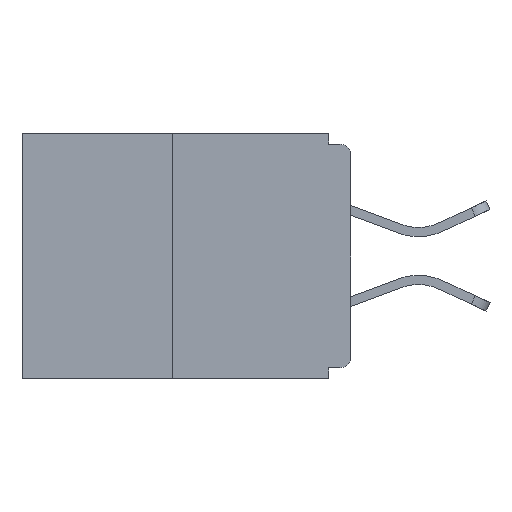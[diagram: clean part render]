
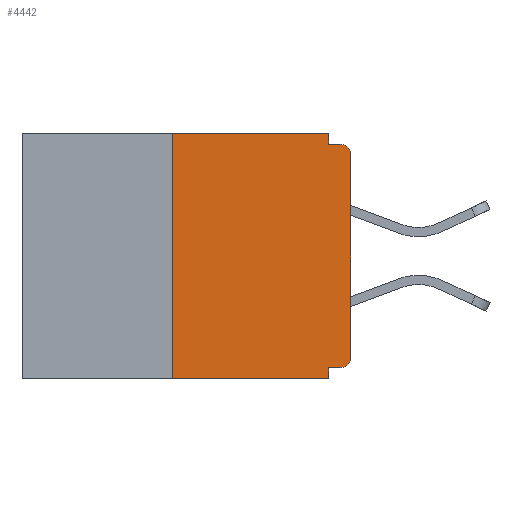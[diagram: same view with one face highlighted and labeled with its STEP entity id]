
A CAD part, left-side view. The second image highlights one B-rep face of the part: STEP entity #4442.
In plain terms, the highlighted planar face has unit normal (-1, 0, 0).
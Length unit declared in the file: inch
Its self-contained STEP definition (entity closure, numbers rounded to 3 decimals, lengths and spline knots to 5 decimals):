
#423 = CARTESIAN_POINT ( 'NONE',  ( 0., 0., -0.015 ) ) ;
#564 = VECTOR ( 'NONE', #16982, 39.37008 ) ;
#706 = DIRECTION ( 'NONE',  ( 1., 0., 0. ) ) ;
#1157 = LINE ( 'NONE', #5550, #12122 ) ;
#1200 = ORIENTED_EDGE ( 'NONE', *, *, #18923, .T. ) ;
#1649 = DIRECTION ( 'NONE',  ( 0., 0., 1. ) ) ;
#1995 = EDGE_LOOP ( 'NONE', ( #3875, #26558, #20291, #4947, #20913, #7943, #1200, #18781, #25721, #5291 ) ) ;
#2291 = DIRECTION ( 'NONE',  ( -1., 0., 0. ) ) ;
#2390 = DIRECTION ( 'NONE',  ( 0., 0., -1. ) ) ;
#3600 = DIRECTION ( 'NONE',  ( 0., -1., 0. ) ) ;
#3779 = CARTESIAN_POINT ( 'NONE',  ( 0., 0.031, -0.343 ) ) ;
#3837 = FACE_OUTER_BOUND ( 'NONE', #1995, .T. ) ;
#3875 = ORIENTED_EDGE ( 'NONE', *, *, #6598, .F. ) ;
#4348 = LINE ( 'NONE', #423, #26550 ) ;
#4442 = ADVANCED_FACE ( 'NONE', ( #3837 ), #6889, .F. ) ;
#4756 = LINE ( 'NONE', #15666, #19653 ) ;
#4944 = DIRECTION ( 'NONE',  ( 0., -1., 0. ) ) ;
#4947 = ORIENTED_EDGE ( 'NONE', *, *, #16179, .F. ) ;
#5106 = EDGE_CURVE ( 'NONE', #24350, #14958, #23606, .T. ) ;
#5291 = ORIENTED_EDGE ( 'NONE', *, *, #20488, .F. ) ;
#5550 = CARTESIAN_POINT ( 'NONE',  ( 0., 0., -0.328 ) ) ;
#5695 = CARTESIAN_POINT ( 'NONE',  ( 0., 0.031, -0.343 ) ) ;
#6598 = EDGE_CURVE ( 'NONE', #8157, #20316, #13883, .T. ) ;
#6620 = CARTESIAN_POINT ( 'NONE',  ( 0., 0., -0.03 ) ) ;
#6793 = EDGE_CURVE ( 'NONE', #8269, #20010, #9901, .T. ) ;
#6889 = PLANE ( 'NONE',  #25837 ) ;
#7943 = ORIENTED_EDGE ( 'NONE', *, *, #6793, .T. ) ;
#8157 = VERTEX_POINT ( 'NONE', #18156 ) ;
#8269 = VERTEX_POINT ( 'NONE', #18789 ) ;
#8326 = VERTEX_POINT ( 'NONE', #19890 ) ;
#8352 = CARTESIAN_POINT ( 'NONE',  ( 0., 0.031, 0. ) ) ;
#9837 = CARTESIAN_POINT ( 'NONE',  ( 0., 0.031, -0.328 ) ) ;
#9865 = VECTOR ( 'NONE', #19667, 39.37008 ) ;
#9901 = CIRCLE ( 'NONE', #16354, 0.015 ) ;
#10922 = CARTESIAN_POINT ( 'NONE',  ( 0., 0.031, 0. ) ) ;
#11319 = CARTESIAN_POINT ( 'NONE',  ( 0., 0., 0. ) ) ;
#12122 = VECTOR ( 'NONE', #13898, 39.37008 ) ;
#12250 = VECTOR ( 'NONE', #3600, 39.37008 ) ;
#12766 = CARTESIAN_POINT ( 'NONE',  ( 0., 0.015, -0.313 ) ) ;
#13309 = DIRECTION ( 'NONE',  ( 0., 0., -1. ) ) ;
#13883 = LINE ( 'NONE', #24522, #12250 ) ;
#13898 = DIRECTION ( 'NONE',  ( 0., 1., 0. ) ) ;
#14958 = VERTEX_POINT ( 'NONE', #15532 ) ;
#15428 = VECTOR ( 'NONE', #18938, 39.37008 ) ;
#15532 = CARTESIAN_POINT ( 'NONE',  ( 0., 0.015, -0.015 ) ) ;
#15666 = CARTESIAN_POINT ( 'NONE',  ( 0., 0.46, -0.343 ) ) ;
#16142 = LINE ( 'NONE', #10922, #564 ) ;
#16179 = EDGE_CURVE ( 'NONE', #23628, #19715, #21429, .T. ) ;
#16354 = AXIS2_PLACEMENT_3D ( 'NONE', #12766, #21296, #2390 ) ;
#16982 = DIRECTION ( 'NONE',  ( 0., 0., -1. ) ) ;
#17023 = EDGE_CURVE ( 'NONE', #8269, #23628, #1157, .T. ) ;
#17207 = DIRECTION ( 'NONE',  ( 0., 0., -1. ) ) ;
#17465 = CARTESIAN_POINT ( 'NONE',  ( 0., 0.031, -0.015 ) ) ;
#17710 = AXIS2_PLACEMENT_3D ( 'NONE', #23404, #2291, #17207 ) ;
#18154 = VERTEX_POINT ( 'NONE', #17465 ) ;
#18156 = CARTESIAN_POINT ( 'NONE',  ( 0., 0.25, 0. ) ) ;
#18781 = ORIENTED_EDGE ( 'NONE', *, *, #5106, .T. ) ;
#18789 = CARTESIAN_POINT ( 'NONE',  ( 0., 0.015, -0.328 ) ) ;
#18923 = EDGE_CURVE ( 'NONE', #20010, #24350, #20152, .T. ) ;
#18938 = DIRECTION ( 'NONE',  ( 0., 0., -1. ) ) ;
#19284 = VECTOR ( 'NONE', #1649, 39.37008 ) ;
#19653 = VECTOR ( 'NONE', #24706, 39.37008 ) ;
#19667 = DIRECTION ( 'NONE',  ( 0., 0., 1. ) ) ;
#19678 = CARTESIAN_POINT ( 'NONE',  ( 0., 0.46, 0. ) ) ;
#19715 = VERTEX_POINT ( 'NONE', #5695 ) ;
#19890 = CARTESIAN_POINT ( 'NONE',  ( 0., 0.25, -0.343 ) ) ;
#19906 = CARTESIAN_POINT ( 'NONE',  ( 0., 0., -0.313 ) ) ;
#20010 = VERTEX_POINT ( 'NONE', #19906 ) ;
#20152 = LINE ( 'NONE', #11319, #9865 ) ;
#20291 = ORIENTED_EDGE ( 'NONE', *, *, #22152, .T. ) ;
#20316 = VERTEX_POINT ( 'NONE', #8352 ) ;
#20488 = EDGE_CURVE ( 'NONE', #20316, #18154, #16142, .T. ) ;
#20632 = LINE ( 'NONE', #21092, #19284 ) ;
#20913 = ORIENTED_EDGE ( 'NONE', *, *, #17023, .F. ) ;
#21092 = CARTESIAN_POINT ( 'NONE',  ( 0., 0.25, 0. ) ) ;
#21296 = DIRECTION ( 'NONE',  ( -1., 0., 0. ) ) ;
#21429 = LINE ( 'NONE', #3779, #15428 ) ;
#22152 = EDGE_CURVE ( 'NONE', #8326, #19715, #4756, .T. ) ;
#23210 = EDGE_CURVE ( 'NONE', #18154, #14958, #4348, .T. ) ;
#23404 = CARTESIAN_POINT ( 'NONE',  ( 0., 0.015, -0.03 ) ) ;
#23606 = CIRCLE ( 'NONE', #17710, 0.015 ) ;
#23628 = VERTEX_POINT ( 'NONE', #9837 ) ;
#24350 = VERTEX_POINT ( 'NONE', #6620 ) ;
#24522 = CARTESIAN_POINT ( 'NONE',  ( 0., 0.46, 0. ) ) ;
#24706 = DIRECTION ( 'NONE',  ( 0., -1., 0. ) ) ;
#25721 = ORIENTED_EDGE ( 'NONE', *, *, #23210, .F. ) ;
#25837 = AXIS2_PLACEMENT_3D ( 'NONE', #19678, #706, #13309 ) ;
#26550 = VECTOR ( 'NONE', #4944, 39.37008 ) ;
#26558 = ORIENTED_EDGE ( 'NONE', *, *, #27375, .F. ) ;
#27375 = EDGE_CURVE ( 'NONE', #8326, #8157, #20632, .T. ) ;
